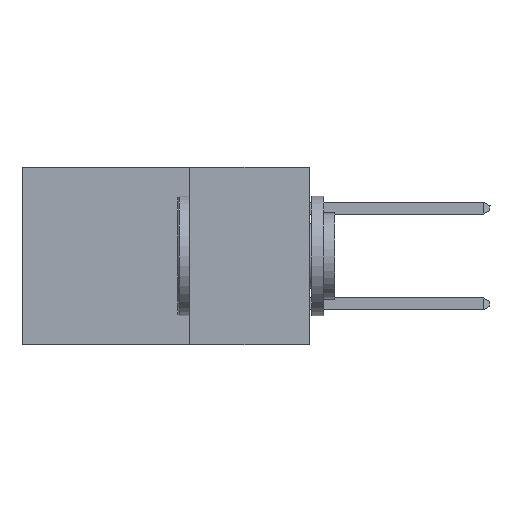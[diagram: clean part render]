
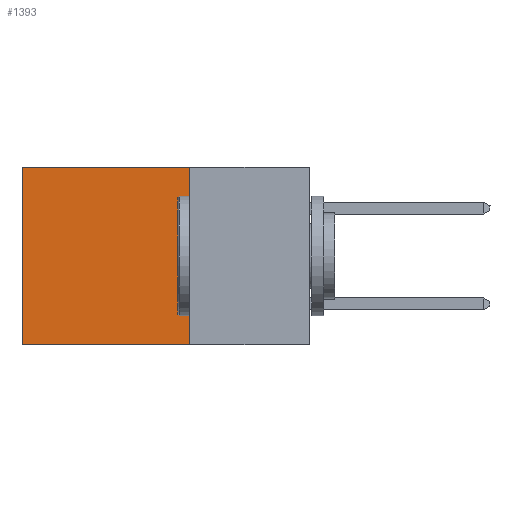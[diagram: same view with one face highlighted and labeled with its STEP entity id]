
A CAD part, left-side view. The second image highlights one B-rep face of the part: STEP entity #1393.
In plain terms, the highlighted planar face has unit normal (-1, 0, 0).
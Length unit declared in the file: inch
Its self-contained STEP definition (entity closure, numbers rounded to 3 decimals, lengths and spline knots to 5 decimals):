
#611 = CARTESIAN_POINT ( 'NONE',  ( 0.2875, 0.25, 0. ) ) ;
#1393 = ADVANCED_FACE ( 'NONE', ( #12118 ), #10830, .F. ) ;
#1482 = DIRECTION ( 'NONE',  ( 1., 0., 0. ) ) ;
#1910 = CARTESIAN_POINT ( 'NONE',  ( 0.2875, 0.6, 0. ) ) ;
#2094 = DIRECTION ( 'NONE',  ( 0., 0., -1. ) ) ;
#2901 = DIRECTION ( 'NONE',  ( 0., 1., 0. ) ) ;
#3314 = AXIS2_PLACEMENT_3D ( 'NONE', #611, #1482, #7843 ) ;
#3372 = CARTESIAN_POINT ( 'NONE',  ( 0.2875, 0.25, -0.37 ) ) ;
#3772 = EDGE_CURVE ( 'NONE', #9322, #12478, #8029, .T. ) ;
#4319 = ORIENTED_EDGE ( 'NONE', *, *, #13149, .T. ) ;
#4549 = ORIENTED_EDGE ( 'NONE', *, *, #5044, .F. ) ;
#5044 = EDGE_CURVE ( 'NONE', #12478, #6832, #11731, .T. ) ;
#5959 = DIRECTION ( 'NONE',  ( 0., 1., 0. ) ) ;
#5995 = EDGE_CURVE ( 'NONE', #9322, #11500, #13154, .T. ) ;
#6832 = VERTEX_POINT ( 'NONE', #13248 ) ;
#7072 = VECTOR ( 'NONE', #2094, 39.37008 ) ;
#7843 = DIRECTION ( 'NONE',  ( 0., 0., -1. ) ) ;
#7995 = ORIENTED_EDGE ( 'NONE', *, *, #3772, .F. ) ;
#8029 = LINE ( 'NONE', #9074, #10282 ) ;
#8305 = VECTOR ( 'NONE', #5959, 39.37008 ) ;
#8323 = CARTESIAN_POINT ( 'NONE',  ( 0.2875, 0.25, 0. ) ) ;
#9074 = CARTESIAN_POINT ( 'NONE',  ( 0.2875, 0.25, 0. ) ) ;
#9118 = CARTESIAN_POINT ( 'NONE',  ( 0.2875, 0.25, 0. ) ) ;
#9226 = DIRECTION ( 'NONE',  ( 0., 0., -1. ) ) ;
#9322 = VERTEX_POINT ( 'NONE', #8323 ) ;
#9612 = VECTOR ( 'NONE', #2901, 39.37008 ) ;
#10282 = VECTOR ( 'NONE', #9226, 39.37008 ) ;
#10830 = PLANE ( 'NONE',  #3314 ) ;
#11500 = VERTEX_POINT ( 'NONE', #1910 ) ;
#11731 = LINE ( 'NONE', #13288, #9612 ) ;
#12118 = FACE_OUTER_BOUND ( 'NONE', #12612, .T. ) ;
#12465 = LINE ( 'NONE', #12679, #7072 ) ;
#12478 = VERTEX_POINT ( 'NONE', #3372 ) ;
#12612 = EDGE_LOOP ( 'NONE', ( #4319, #4549, #7995, #13011 ) ) ;
#12679 = CARTESIAN_POINT ( 'NONE',  ( 0.2875, 0.6, 0. ) ) ;
#13011 = ORIENTED_EDGE ( 'NONE', *, *, #5995, .T. ) ;
#13149 = EDGE_CURVE ( 'NONE', #11500, #6832, #12465, .T. ) ;
#13154 = LINE ( 'NONE', #9118, #8305 ) ;
#13248 = CARTESIAN_POINT ( 'NONE',  ( 0.2875, 0.6, -0.37 ) ) ;
#13288 = CARTESIAN_POINT ( 'NONE',  ( 0.2875, 0.25, -0.37 ) ) ;
